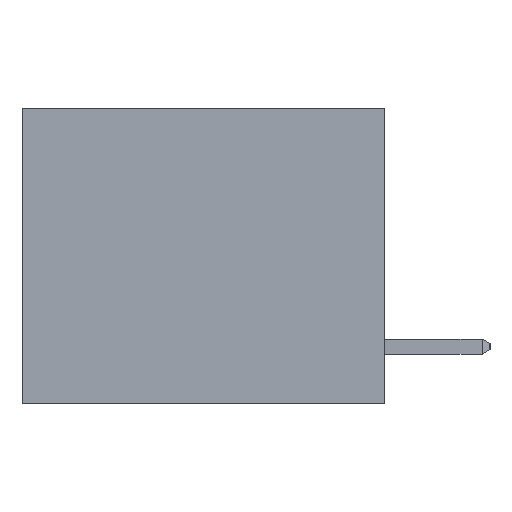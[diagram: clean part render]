
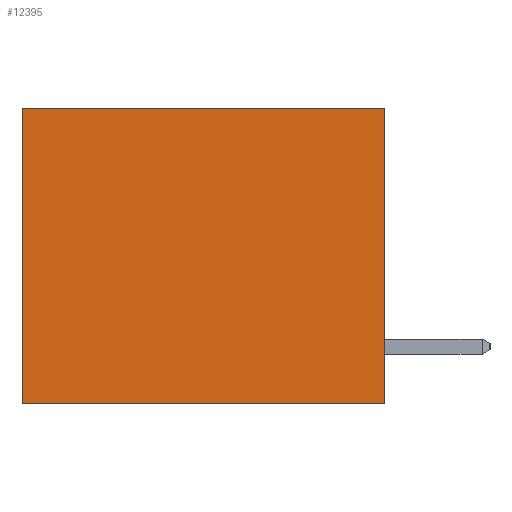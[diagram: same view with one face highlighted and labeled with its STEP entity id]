
A CAD part, left-side view. The second image highlights one B-rep face of the part: STEP entity #12395.
In plain terms, the highlighted planar face has unit normal (-1, 0, 0).
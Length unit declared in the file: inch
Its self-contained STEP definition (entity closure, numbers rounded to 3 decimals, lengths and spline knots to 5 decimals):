
#991 = VERTEX_POINT ( 'NONE', #7618 ) ;
#3397 = DIRECTION ( 'NONE',  ( 0., 1., 0. ) ) ;
#3544 = LINE ( 'NONE', #7745, #17990 ) ;
#3660 = EDGE_CURVE ( 'NONE', #20169, #10565, #3544, .T. ) ;
#3915 = EDGE_CURVE ( 'NONE', #20169, #15240, #9258, .T. ) ;
#4440 = ORIENTED_EDGE ( 'NONE', *, *, #3915, .T. ) ;
#5226 = CARTESIAN_POINT ( 'NONE',  ( 0.3165, 0., 0. ) ) ;
#5241 = ORIENTED_EDGE ( 'NONE', *, *, #13381, .T. ) ;
#6245 = DIRECTION ( 'NONE',  ( 0., 0., -1. ) ) ;
#6578 = CARTESIAN_POINT ( 'NONE',  ( 0.3165, 0.6, 0. ) ) ;
#7550 = ORIENTED_EDGE ( 'NONE', *, *, #15589, .F. ) ;
#7618 = CARTESIAN_POINT ( 'NONE',  ( 0.3165, 0.6, -0.49 ) ) ;
#7745 = CARTESIAN_POINT ( 'NONE',  ( 0.3165, 0., -0.49 ) ) ;
#7755 = AXIS2_PLACEMENT_3D ( 'NONE', #9732, #21924, #18957 ) ;
#8895 = EDGE_LOOP ( 'NONE', ( #5241, #7550, #20446, #4440 ) ) ;
#9258 = LINE ( 'NONE', #5226, #14443 ) ;
#9732 = CARTESIAN_POINT ( 'NONE',  ( 0.3165, 0., -0.49 ) ) ;
#10002 = LINE ( 'NONE', #15507, #18727 ) ;
#10565 = VERTEX_POINT ( 'NONE', #15427 ) ;
#12395 = ADVANCED_FACE ( 'NONE', ( #21852 ), #20189, .F. ) ;
#12583 = LINE ( 'NONE', #12730, #18026 ) ;
#12730 = CARTESIAN_POINT ( 'NONE',  ( 0.3165, 0.6, -0.49 ) ) ;
#12975 = CARTESIAN_POINT ( 'NONE',  ( 0.3165, 0., 0. ) ) ;
#13381 = EDGE_CURVE ( 'NONE', #15240, #991, #12583, .T. ) ;
#14443 = VECTOR ( 'NONE', #17415, 39.37008 ) ;
#15240 = VERTEX_POINT ( 'NONE', #6578 ) ;
#15427 = CARTESIAN_POINT ( 'NONE',  ( 0.3165, 0., -0.49 ) ) ;
#15507 = CARTESIAN_POINT ( 'NONE',  ( 0.3165, 0., -0.49 ) ) ;
#15589 = EDGE_CURVE ( 'NONE', #10565, #991, #10002, .T. ) ;
#17415 = DIRECTION ( 'NONE',  ( 0., 1., 0. ) ) ;
#17990 = VECTOR ( 'NONE', #20093, 39.37008 ) ;
#18026 = VECTOR ( 'NONE', #6245, 39.37008 ) ;
#18727 = VECTOR ( 'NONE', #3397, 39.37008 ) ;
#18957 = DIRECTION ( 'NONE',  ( 0., 0., -1. ) ) ;
#20093 = DIRECTION ( 'NONE',  ( 0., 0., -1. ) ) ;
#20169 = VERTEX_POINT ( 'NONE', #12975 ) ;
#20189 = PLANE ( 'NONE',  #7755 ) ;
#20446 = ORIENTED_EDGE ( 'NONE', *, *, #3660, .F. ) ;
#21852 = FACE_OUTER_BOUND ( 'NONE', #8895, .T. ) ;
#21924 = DIRECTION ( 'NONE',  ( 1., 0., 0. ) ) ;
